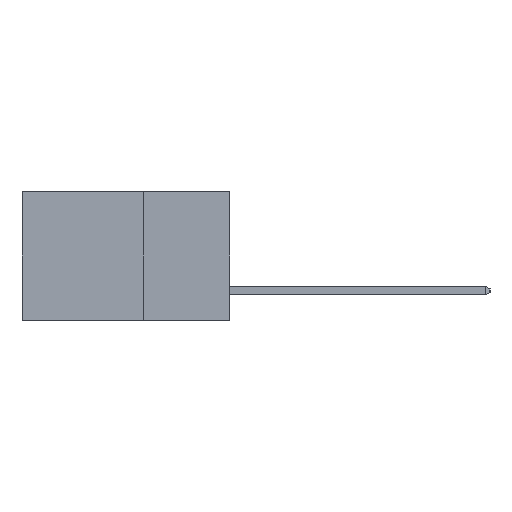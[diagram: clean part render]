
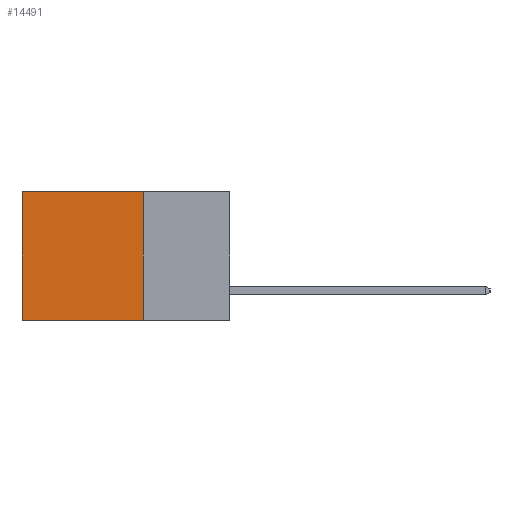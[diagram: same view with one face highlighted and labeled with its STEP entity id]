
A CAD part, left-side view. The second image highlights one B-rep face of the part: STEP entity #14491.
In plain terms, the highlighted planar face has unit normal (-1, 0, 0).
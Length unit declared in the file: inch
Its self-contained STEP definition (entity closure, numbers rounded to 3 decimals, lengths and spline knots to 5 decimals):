
#1734 = VERTEX_POINT ( 'NONE', #16992 ) ;
#1736 = EDGE_CURVE ( 'NONE', #20862, #1734, #8742, .T. ) ;
#3046 = VERTEX_POINT ( 'NONE', #15201 ) ;
#3535 = DIRECTION ( 'NONE',  ( 0., 1., 0. ) ) ;
#3929 = VECTOR ( 'NONE', #3535, 39.37008 ) ;
#4166 = CARTESIAN_POINT ( 'NONE',  ( 0.298, 0.6, 0. ) ) ;
#5675 = EDGE_CURVE ( 'NONE', #20862, #8100, #9839, .T. ) ;
#6635 = EDGE_CURVE ( 'NONE', #1734, #3046, #10008, .T. ) ;
#7440 = CARTESIAN_POINT ( 'NONE',  ( 0.298, 0.25, 0. ) ) ;
#7751 = PLANE ( 'NONE',  #9738 ) ;
#8100 = VERTEX_POINT ( 'NONE', #26264 ) ;
#8155 = CARTESIAN_POINT ( 'NONE',  ( 0.298, 0.25, 0. ) ) ;
#8742 = LINE ( 'NONE', #8155, #19834 ) ;
#9738 = AXIS2_PLACEMENT_3D ( 'NONE', #18828, #23289, #9974 ) ;
#9839 = LINE ( 'NONE', #23356, #3929 ) ;
#9908 = ORIENTED_EDGE ( 'NONE', *, *, #5675, .T. ) ;
#9974 = DIRECTION ( 'NONE',  ( 0., 0., -1. ) ) ;
#10008 = LINE ( 'NONE', #25859, #21119 ) ;
#12003 = VECTOR ( 'NONE', #15265, 39.37008 ) ;
#12160 = ORIENTED_EDGE ( 'NONE', *, *, #1736, .F. ) ;
#14491 = ADVANCED_FACE ( 'NONE', ( #21412 ), #7751, .F. ) ;
#15201 = CARTESIAN_POINT ( 'NONE',  ( 0.298, 0.6, -0.37 ) ) ;
#15265 = DIRECTION ( 'NONE',  ( 0., 0., -1. ) ) ;
#16209 = EDGE_LOOP ( 'NONE', ( #28465, #23408, #12160, #9908 ) ) ;
#16992 = CARTESIAN_POINT ( 'NONE',  ( 0.298, 0.25, -0.37 ) ) ;
#17092 = DIRECTION ( 'NONE',  ( 0., 1., 0. ) ) ;
#18452 = EDGE_CURVE ( 'NONE', #8100, #3046, #24484, .T. ) ;
#18828 = CARTESIAN_POINT ( 'NONE',  ( 0.298, 0.25, 0. ) ) ;
#19834 = VECTOR ( 'NONE', #23678, 39.37008 ) ;
#20862 = VERTEX_POINT ( 'NONE', #7440 ) ;
#21119 = VECTOR ( 'NONE', #17092, 39.37008 ) ;
#21412 = FACE_OUTER_BOUND ( 'NONE', #16209, .T. ) ;
#23289 = DIRECTION ( 'NONE',  ( 1., 0., 0. ) ) ;
#23356 = CARTESIAN_POINT ( 'NONE',  ( 0.298, 0.25, 0. ) ) ;
#23408 = ORIENTED_EDGE ( 'NONE', *, *, #6635, .F. ) ;
#23678 = DIRECTION ( 'NONE',  ( 0., 0., -1. ) ) ;
#24484 = LINE ( 'NONE', #4166, #12003 ) ;
#25859 = CARTESIAN_POINT ( 'NONE',  ( 0.298, 0.25, -0.37 ) ) ;
#26264 = CARTESIAN_POINT ( 'NONE',  ( 0.298, 0.6, 0. ) ) ;
#28465 = ORIENTED_EDGE ( 'NONE', *, *, #18452, .T. ) ;
